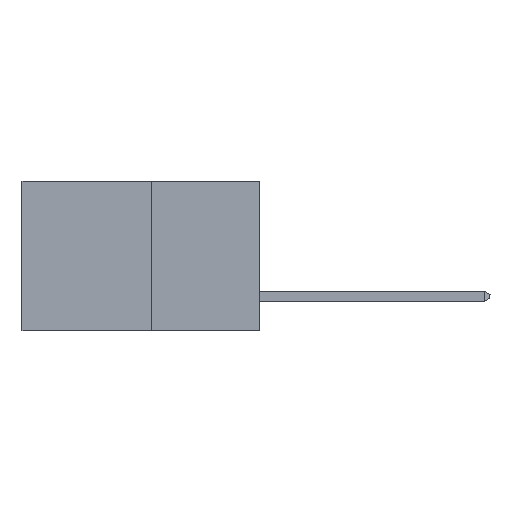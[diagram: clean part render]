
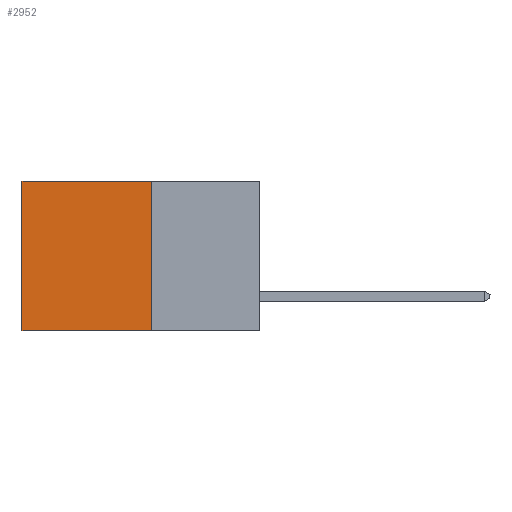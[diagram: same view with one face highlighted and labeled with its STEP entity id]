
A CAD part, left-side view. The second image highlights one B-rep face of the part: STEP entity #2952.
In plain terms, the highlighted planar face has unit normal (-1, 0, 0).
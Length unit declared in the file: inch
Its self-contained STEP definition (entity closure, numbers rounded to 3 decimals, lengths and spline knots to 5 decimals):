
#278 = EDGE_CURVE ( 'NONE', #10718, #7654, #8455, .T. ) ;
#548 = EDGE_CURVE ( 'NONE', #7654, #7991, #14121, .T. ) ;
#923 = CARTESIAN_POINT ( 'NONE',  ( 0.277, 0.59, -0.37 ) ) ;
#1073 = CARTESIAN_POINT ( 'NONE',  ( 0.277, 0.59, 0. ) ) ;
#1127 = DIRECTION ( 'NONE',  ( 0., 0., -1. ) ) ;
#1141 = EDGE_CURVE ( 'NONE', #10718, #14005, #11386, .T. ) ;
#1670 = CARTESIAN_POINT ( 'NONE',  ( 0.277, 0.59, -0.37 ) ) ;
#1964 = FACE_OUTER_BOUND ( 'NONE', #8955, .T. ) ;
#2521 = LINE ( 'NONE', #8606, #8783 ) ;
#2952 = ADVANCED_FACE ( 'NONE', ( #1964 ), #9475, .F. ) ;
#3854 = ORIENTED_EDGE ( 'NONE', *, *, #278, .T. ) ;
#4010 = CARTESIAN_POINT ( 'NONE',  ( 0.277, 0.27, 0. ) ) ;
#4338 = ORIENTED_EDGE ( 'NONE', *, *, #7649, .F. ) ;
#4750 = VECTOR ( 'NONE', #1127, 39.37008 ) ;
#5462 = ORIENTED_EDGE ( 'NONE', *, *, #548, .T. ) ;
#7649 = EDGE_CURVE ( 'NONE', #14005, #7991, #2521, .T. ) ;
#7654 = VERTEX_POINT ( 'NONE', #1073 ) ;
#7991 = VERTEX_POINT ( 'NONE', #1670 ) ;
#8455 = LINE ( 'NONE', #14371, #14514 ) ;
#8606 = CARTESIAN_POINT ( 'NONE',  ( 0.277, 0.27, -0.37 ) ) ;
#8775 = CARTESIAN_POINT ( 'NONE',  ( 0.277, 0.27, -0.37 ) ) ;
#8783 = VECTOR ( 'NONE', #9856, 39.37008 ) ;
#8955 = EDGE_LOOP ( 'NONE', ( #5462, #4338, #15140, #3854 ) ) ;
#9330 = DIRECTION ( 'NONE',  ( 0., 0., -1. ) ) ;
#9381 = DIRECTION ( 'NONE',  ( 1., 0., 0. ) ) ;
#9404 = DIRECTION ( 'NONE',  ( 0., 0., -1. ) ) ;
#9475 = PLANE ( 'NONE',  #11746 ) ;
#9856 = DIRECTION ( 'NONE',  ( 0., 1., 0. ) ) ;
#9942 = CARTESIAN_POINT ( 'NONE',  ( 0.277, 0.27, -0.37 ) ) ;
#10718 = VERTEX_POINT ( 'NONE', #4010 ) ;
#11386 = LINE ( 'NONE', #8775, #14550 ) ;
#11525 = DIRECTION ( 'NONE',  ( 0., 1., 0. ) ) ;
#11746 = AXIS2_PLACEMENT_3D ( 'NONE', #9942, #9381, #9330 ) ;
#14005 = VERTEX_POINT ( 'NONE', #15373 ) ;
#14121 = LINE ( 'NONE', #923, #4750 ) ;
#14371 = CARTESIAN_POINT ( 'NONE',  ( 0.277, 0.27, 0. ) ) ;
#14514 = VECTOR ( 'NONE', #11525, 39.37008 ) ;
#14550 = VECTOR ( 'NONE', #9404, 39.37008 ) ;
#15140 = ORIENTED_EDGE ( 'NONE', *, *, #1141, .F. ) ;
#15373 = CARTESIAN_POINT ( 'NONE',  ( 0.277, 0.27, -0.37 ) ) ;
